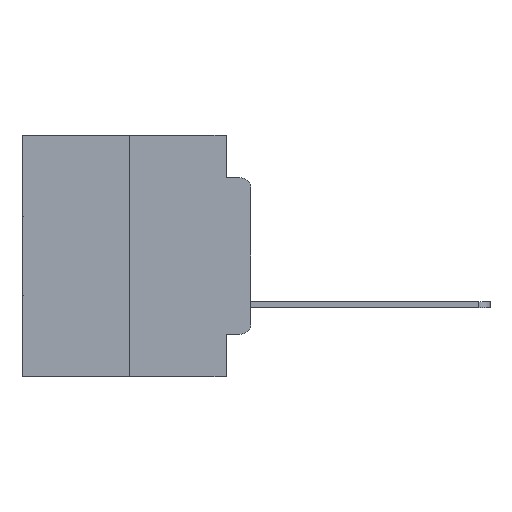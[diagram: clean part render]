
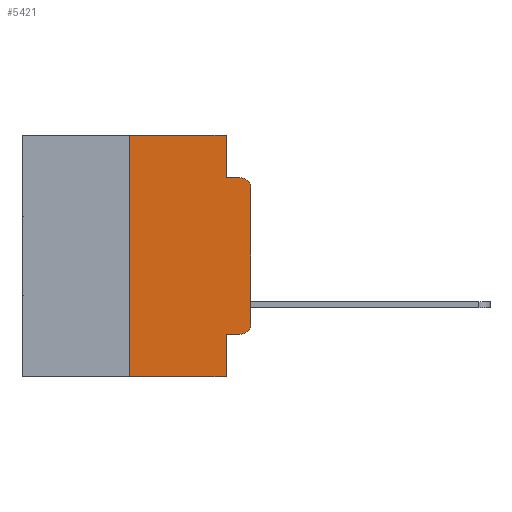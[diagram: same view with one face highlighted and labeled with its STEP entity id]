
A CAD part, left-side view. The second image highlights one B-rep face of the part: STEP entity #5421.
In plain terms, the highlighted planar face has unit normal (-1, 0, 0).
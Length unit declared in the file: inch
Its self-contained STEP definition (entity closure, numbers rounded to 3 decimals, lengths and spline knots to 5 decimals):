
#11 = CARTESIAN_POINT ( 'NONE',  ( 0., 0.02, -0.1085 ) ) ;
#350 = LINE ( 'NONE', #24387, #5288 ) ;
#476 = DIRECTION ( 'NONE',  ( 0., -1., 0. ) ) ;
#564 = ORIENTED_EDGE ( 'NONE', *, *, #19296, .T. ) ;
#822 = CARTESIAN_POINT ( 'NONE',  ( 0., 0.051, 0. ) ) ;
#1970 = VERTEX_POINT ( 'NONE', #5321 ) ;
#2073 = CARTESIAN_POINT ( 'NONE',  ( 0., 0.051, -0.4115 ) ) ;
#2408 = DIRECTION ( 'NONE',  ( 0., 0., -1. ) ) ;
#2465 = DIRECTION ( 'NONE',  ( 1., 0., 0. ) ) ;
#2513 = LINE ( 'NONE', #2073, #20202 ) ;
#2888 = LINE ( 'NONE', #16232, #26508 ) ;
#3645 = ORIENTED_EDGE ( 'NONE', *, *, #24928, .T. ) ;
#3933 = LINE ( 'NONE', #9434, #20807 ) ;
#3983 = ORIENTED_EDGE ( 'NONE', *, *, #11102, .T. ) ;
#4746 = EDGE_CURVE ( 'NONE', #8073, #18789, #2888, .T. ) ;
#5288 = VECTOR ( 'NONE', #28862, 39.37008 ) ;
#5321 = CARTESIAN_POINT ( 'NONE',  ( 0., 0.25, 0. ) ) ;
#5421 = ADVANCED_FACE ( 'NONE', ( #9511 ), #16406, .F. ) ;
#5820 = CARTESIAN_POINT ( 'NONE',  ( 0., 0.02, -0.0885 ) ) ;
#6061 = CARTESIAN_POINT ( 'NONE',  ( 0., 0., -0.3915 ) ) ;
#6313 = VERTEX_POINT ( 'NONE', #6766 ) ;
#6659 = VERTEX_POINT ( 'NONE', #822 ) ;
#6766 = CARTESIAN_POINT ( 'NONE',  ( 0., 0.02, -0.4115 ) ) ;
#6946 = DIRECTION ( 'NONE',  ( 0., -1., 0. ) ) ;
#8073 = VERTEX_POINT ( 'NONE', #17956 ) ;
#8103 = CARTESIAN_POINT ( 'NONE',  ( 0., 0.051, 0. ) ) ;
#9151 = ORIENTED_EDGE ( 'NONE', *, *, #13218, .F. ) ;
#9433 = CARTESIAN_POINT ( 'NONE',  ( 0., 0.051, -0.0885 ) ) ;
#9434 = CARTESIAN_POINT ( 'NONE',  ( 0., 0.25, 0. ) ) ;
#9511 = FACE_OUTER_BOUND ( 'NONE', #13205, .T. ) ;
#9514 = VERTEX_POINT ( 'NONE', #5820 ) ;
#10251 = ORIENTED_EDGE ( 'NONE', *, *, #21340, .F. ) ;
#11017 = CIRCLE ( 'NONE', #22263, 0.02 ) ;
#11102 = EDGE_CURVE ( 'NONE', #18995, #22175, #350, .T. ) ;
#11240 = CARTESIAN_POINT ( 'NONE',  ( 0., 0.02, -0.3915 ) ) ;
#11788 = CARTESIAN_POINT ( 'NONE',  ( 0., 0.051, 0. ) ) ;
#12402 = CARTESIAN_POINT ( 'NONE',  ( 0., 0.051, -0.4115 ) ) ;
#12675 = CARTESIAN_POINT ( 'NONE',  ( 0., 0.051, -0.0885 ) ) ;
#13205 = EDGE_LOOP ( 'NONE', ( #3983, #564, #9151, #22605, #19480, #10251, #22974, #18428, #3645, #16688 ) ) ;
#13218 = EDGE_CURVE ( 'NONE', #17567, #9514, #23765, .T. ) ;
#13549 = DIRECTION ( 'NONE',  ( 0., 0., -1. ) ) ;
#14793 = CARTESIAN_POINT ( 'NONE',  ( 0., 0., -0.1085 ) ) ;
#14892 = DIRECTION ( 'NONE',  ( 0., 0., -1. ) ) ;
#16232 = CARTESIAN_POINT ( 'NONE',  ( 0., 0.473, -0.5 ) ) ;
#16347 = DIRECTION ( 'NONE',  ( -1., 0., 0. ) ) ;
#16406 = PLANE ( 'NONE',  #23184 ) ;
#16688 = ORIENTED_EDGE ( 'NONE', *, *, #17402, .T. ) ;
#17271 = DIRECTION ( 'NONE',  ( 0., -1., 0. ) ) ;
#17402 = EDGE_CURVE ( 'NONE', #6313, #18995, #11017, .T. ) ;
#17567 = VERTEX_POINT ( 'NONE', #9433 ) ;
#17956 = CARTESIAN_POINT ( 'NONE',  ( 0., 0.25, -0.5 ) ) ;
#18428 = ORIENTED_EDGE ( 'NONE', *, *, #26405, .F. ) ;
#18498 = VECTOR ( 'NONE', #23140, 39.37008 ) ;
#18591 = DIRECTION ( 'NONE',  ( 0., 0., 1. ) ) ;
#18671 = DIRECTION ( 'NONE',  ( 0., 0., -1. ) ) ;
#18789 = VERTEX_POINT ( 'NONE', #18952 ) ;
#18952 = CARTESIAN_POINT ( 'NONE',  ( 0., 0.051, -0.5 ) ) ;
#18995 = VERTEX_POINT ( 'NONE', #6061 ) ;
#19070 = CARTESIAN_POINT ( 'NONE',  ( 0., 0.473, 0. ) ) ;
#19296 = EDGE_CURVE ( 'NONE', #22175, #9514, #25337, .T. ) ;
#19480 = ORIENTED_EDGE ( 'NONE', *, *, #28453, .F. ) ;
#20202 = VECTOR ( 'NONE', #6946, 39.37008 ) ;
#20807 = VECTOR ( 'NONE', #18591, 39.37008 ) ;
#21340 = EDGE_CURVE ( 'NONE', #8073, #1970, #3933, .T. ) ;
#22175 = VERTEX_POINT ( 'NONE', #14793 ) ;
#22263 = AXIS2_PLACEMENT_3D ( 'NONE', #11240, #27009, #13549 ) ;
#22605 = ORIENTED_EDGE ( 'NONE', *, *, #24343, .F. ) ;
#22641 = VECTOR ( 'NONE', #476, 39.37008 ) ;
#22974 = ORIENTED_EDGE ( 'NONE', *, *, #4746, .T. ) ;
#23069 = CARTESIAN_POINT ( 'NONE',  ( 0., 0.473, 0. ) ) ;
#23140 = DIRECTION ( 'NONE',  ( 0., 0., -1. ) ) ;
#23184 = AXIS2_PLACEMENT_3D ( 'NONE', #23069, #2465, #18671 ) ;
#23355 = LINE ( 'NONE', #19070, #22641 ) ;
#23765 = LINE ( 'NONE', #12675, #28973 ) ;
#24343 = EDGE_CURVE ( 'NONE', #6659, #17567, #24455, .T. ) ;
#24387 = CARTESIAN_POINT ( 'NONE',  ( 0., 0., 0. ) ) ;
#24455 = LINE ( 'NONE', #11788, #18498 ) ;
#24928 = EDGE_CURVE ( 'NONE', #25818, #6313, #2513, .T. ) ;
#25287 = DIRECTION ( 'NONE',  ( 0., -1., 0. ) ) ;
#25337 = CIRCLE ( 'NONE', #29382, 0.02 ) ;
#25734 = VECTOR ( 'NONE', #14892, 39.37008 ) ;
#25818 = VERTEX_POINT ( 'NONE', #12402 ) ;
#26405 = EDGE_CURVE ( 'NONE', #25818, #18789, #27121, .T. ) ;
#26508 = VECTOR ( 'NONE', #25287, 39.37008 ) ;
#27009 = DIRECTION ( 'NONE',  ( -1., 0., 0. ) ) ;
#27121 = LINE ( 'NONE', #8103, #25734 ) ;
#28453 = EDGE_CURVE ( 'NONE', #1970, #6659, #23355, .T. ) ;
#28862 = DIRECTION ( 'NONE',  ( 0., 0., 1. ) ) ;
#28973 = VECTOR ( 'NONE', #17271, 39.37008 ) ;
#29382 = AXIS2_PLACEMENT_3D ( 'NONE', #11, #16347, #2408 ) ;
